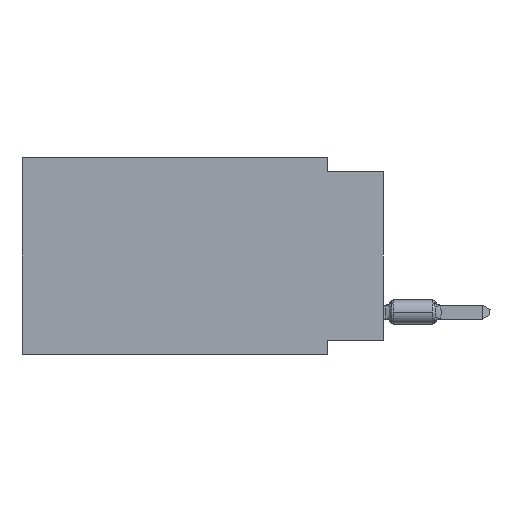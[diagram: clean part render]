
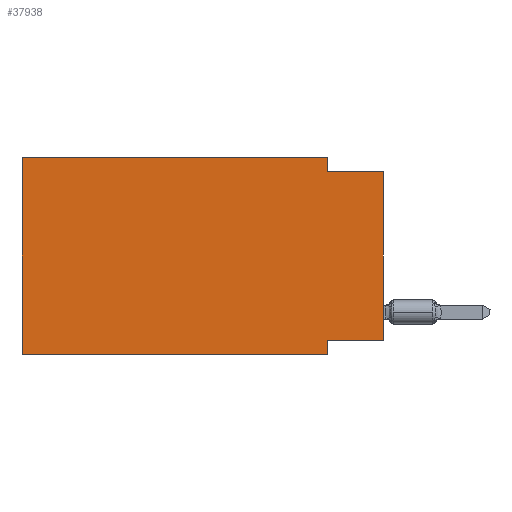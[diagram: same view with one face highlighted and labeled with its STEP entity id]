
A CAD part, left-side view. The second image highlights one B-rep face of the part: STEP entity #37938.
In plain terms, the highlighted planar face has unit normal (-1, 0, 0).
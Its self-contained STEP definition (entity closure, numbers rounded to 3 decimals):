
#530 = DIRECTION ( 'NONE',  ( 0., -1., 0. ) ) ;
#939 = AXIS2_PLACEMENT_3D ( 'NONE', #46598, #2076, #20367 ) ;
#994 = CARTESIAN_POINT ( 'NONE',  ( 0., 2.54, -8.89 ) ) ;
#1750 = VECTOR ( 'NONE', #54959, 1000. ) ;
#1774 = PLANE ( 'NONE',  #939 ) ;
#1828 = VERTEX_POINT ( 'NONE', #31033 ) ;
#2076 = DIRECTION ( 'NONE',  ( 1., 0., 0. ) ) ;
#2270 = EDGE_CURVE ( 'NONE', #46258, #3270, #41236, .T. ) ;
#2788 = EDGE_CURVE ( 'NONE', #29249, #3270, #11611, .T. ) ;
#3270 = VERTEX_POINT ( 'NONE', #43098 ) ;
#3911 = CARTESIAN_POINT ( 'NONE',  ( 0., 0., 0. ) ) ;
#7165 = DIRECTION ( 'NONE',  ( 0., 0., 1. ) ) ;
#7704 = EDGE_CURVE ( 'NONE', #51302, #34408, #13395, .T. ) ;
#7764 = EDGE_CURVE ( 'NONE', #45784, #12311, #9245, .T. ) ;
#9245 = LINE ( 'NONE', #13670, #21787 ) ;
#9838 = DIRECTION ( 'NONE',  ( 0., 0., -1. ) ) ;
#10361 = EDGE_LOOP ( 'NONE', ( #38006, #46568, #32697, #20649, #48863, #47055, #14638, #30043 ) ) ;
#11611 = LINE ( 'NONE', #3911, #34503 ) ;
#12311 = VERTEX_POINT ( 'NONE', #57007 ) ;
#13395 = LINE ( 'NONE', #994, #45298 ) ;
#13670 = CARTESIAN_POINT ( 'NONE',  ( 0., 16.383, 0. ) ) ;
#14638 = ORIENTED_EDGE ( 'NONE', *, *, #7704, .F. ) ;
#15534 = EDGE_CURVE ( 'NONE', #12311, #1828, #18899, .T. ) ;
#15875 = LINE ( 'NONE', #28858, #47517 ) ;
#18541 = CARTESIAN_POINT ( 'NONE',  ( 0., 0., -0.635 ) ) ;
#18899 = LINE ( 'NONE', #50434, #37259 ) ;
#19232 = EDGE_CURVE ( 'NONE', #1828, #46258, #52678, .T. ) ;
#20367 = DIRECTION ( 'NONE',  ( 0., 0., -1. ) ) ;
#20649 = ORIENTED_EDGE ( 'NONE', *, *, #15534, .F. ) ;
#21787 = VECTOR ( 'NONE', #45815, 1000. ) ;
#23462 = CARTESIAN_POINT ( 'NONE',  ( 0., 16.383, -8.89 ) ) ;
#26086 = DIRECTION ( 'NONE',  ( 0., 1., 0. ) ) ;
#28858 = CARTESIAN_POINT ( 'NONE',  ( 0., 0., -8.255 ) ) ;
#29249 = VERTEX_POINT ( 'NONE', #35022 ) ;
#30043 = ORIENTED_EDGE ( 'NONE', *, *, #54851, .F. ) ;
#31033 = CARTESIAN_POINT ( 'NONE',  ( 0., 2.54, 0. ) ) ;
#32697 = ORIENTED_EDGE ( 'NONE', *, *, #19232, .F. ) ;
#34408 = VERTEX_POINT ( 'NONE', #49222 ) ;
#34503 = VECTOR ( 'NONE', #7165, 1000. ) ;
#35022 = CARTESIAN_POINT ( 'NONE',  ( 0., 0., -8.255 ) ) ;
#35397 = EDGE_CURVE ( 'NONE', #45784, #34408, #37553, .T. ) ;
#36645 = CARTESIAN_POINT ( 'NONE',  ( 0., 2.54, -8.255 ) ) ;
#36961 = CARTESIAN_POINT ( 'NONE',  ( 0., 16.383, -8.89 ) ) ;
#37259 = VECTOR ( 'NONE', #42484, 1000. ) ;
#37553 = LINE ( 'NONE', #36961, #1750 ) ;
#37938 = ADVANCED_FACE ( 'NONE', ( #42777 ), #1774, .F. ) ;
#38006 = ORIENTED_EDGE ( 'NONE', *, *, #2788, .T. ) ;
#41236 = LINE ( 'NONE', #18541, #48592 ) ;
#42484 = DIRECTION ( 'NONE',  ( 0., -1., 0. ) ) ;
#42777 = FACE_OUTER_BOUND ( 'NONE', #10361, .T. ) ;
#43098 = CARTESIAN_POINT ( 'NONE',  ( 0., 0., -0.635 ) ) ;
#43132 = VECTOR ( 'NONE', #57677, 1000. ) ;
#45298 = VECTOR ( 'NONE', #9838, 1000. ) ;
#45784 = VERTEX_POINT ( 'NONE', #23462 ) ;
#45815 = DIRECTION ( 'NONE',  ( 0., 0., 1. ) ) ;
#46258 = VERTEX_POINT ( 'NONE', #57676 ) ;
#46568 = ORIENTED_EDGE ( 'NONE', *, *, #2270, .F. ) ;
#46598 = CARTESIAN_POINT ( 'NONE',  ( 0., 16.383, 0. ) ) ;
#47055 = ORIENTED_EDGE ( 'NONE', *, *, #35397, .T. ) ;
#47517 = VECTOR ( 'NONE', #26086, 1000. ) ;
#48592 = VECTOR ( 'NONE', #530, 1000. ) ;
#48863 = ORIENTED_EDGE ( 'NONE', *, *, #7764, .F. ) ;
#49222 = CARTESIAN_POINT ( 'NONE',  ( 0., 2.54, -8.89 ) ) ;
#50434 = CARTESIAN_POINT ( 'NONE',  ( 0., 16.383, 0. ) ) ;
#51302 = VERTEX_POINT ( 'NONE', #36645 ) ;
#52107 = CARTESIAN_POINT ( 'NONE',  ( 0., 2.54, 0. ) ) ;
#52678 = LINE ( 'NONE', #52107, #43132 ) ;
#54851 = EDGE_CURVE ( 'NONE', #29249, #51302, #15875, .T. ) ;
#54959 = DIRECTION ( 'NONE',  ( 0., -1., 0. ) ) ;
#57007 = CARTESIAN_POINT ( 'NONE',  ( 0., 16.383, 0. ) ) ;
#57676 = CARTESIAN_POINT ( 'NONE',  ( 0., 2.54, -0.635 ) ) ;
#57677 = DIRECTION ( 'NONE',  ( 0., 0., -1. ) ) ;
